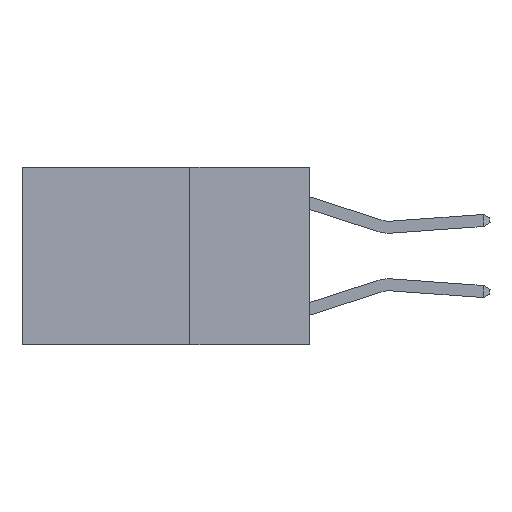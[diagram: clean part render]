
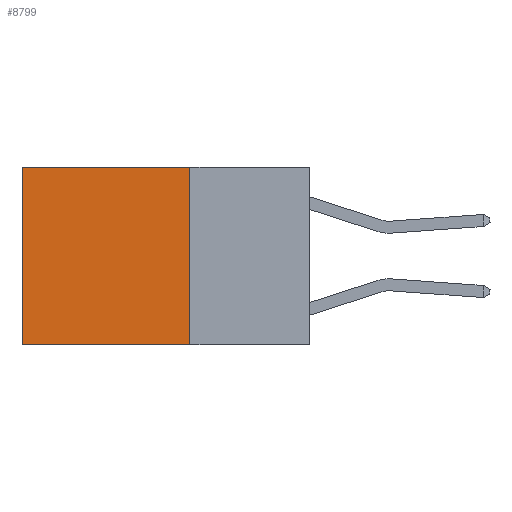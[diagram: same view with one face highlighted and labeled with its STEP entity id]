
A CAD part, left-side view. The second image highlights one B-rep face of the part: STEP entity #8799.
In plain terms, the highlighted planar face has unit normal (-1, 0, 0).
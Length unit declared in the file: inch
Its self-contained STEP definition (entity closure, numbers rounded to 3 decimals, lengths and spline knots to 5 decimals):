
#85 = ORIENTED_EDGE ( 'NONE', *, *, #1875, .F. ) ;
#963 = EDGE_CURVE ( 'NONE', #2235, #10444, #7236, .T. ) ;
#1875 = EDGE_CURVE ( 'NONE', #7877, #9755, #11947, .T. ) ;
#2063 = CARTESIAN_POINT ( 'NONE',  ( 0.2625, 0.25, 0. ) ) ;
#2235 = VERTEX_POINT ( 'NONE', #2063 ) ;
#2325 = CARTESIAN_POINT ( 'NONE',  ( 0.2625, 0.6, 0. ) ) ;
#3288 = DIRECTION ( 'NONE',  ( 0., 1., 0. ) ) ;
#3861 = AXIS2_PLACEMENT_3D ( 'NONE', #6731, #15380, #10451 ) ;
#4189 = CARTESIAN_POINT ( 'NONE',  ( 0.2625, 0.25, 0. ) ) ;
#5279 = DIRECTION ( 'NONE',  ( 0., 0., -1. ) ) ;
#5833 = DIRECTION ( 'NONE',  ( 0., 0., -1. ) ) ;
#6412 = CARTESIAN_POINT ( 'NONE',  ( 0.2625, 0.25, -0.37 ) ) ;
#6438 = CARTESIAN_POINT ( 'NONE',  ( 0.2625, 0.6, -0.37 ) ) ;
#6731 = CARTESIAN_POINT ( 'NONE',  ( 0.2625, 0.25, 0. ) ) ;
#6911 = VECTOR ( 'NONE', #3288, 39.37008 ) ;
#6963 = CARTESIAN_POINT ( 'NONE',  ( 0.2625, 0.25, -0.37 ) ) ;
#7236 = LINE ( 'NONE', #7550, #7665 ) ;
#7550 = CARTESIAN_POINT ( 'NONE',  ( 0.2625, 0.25, 0. ) ) ;
#7665 = VECTOR ( 'NONE', #8427, 39.37008 ) ;
#7877 = VERTEX_POINT ( 'NONE', #6412 ) ;
#8038 = CARTESIAN_POINT ( 'NONE',  ( 0.2625, 0.6, 0. ) ) ;
#8427 = DIRECTION ( 'NONE',  ( 0., 1., 0. ) ) ;
#8585 = EDGE_CURVE ( 'NONE', #2235, #7877, #15173, .T. ) ;
#8799 = ADVANCED_FACE ( 'NONE', ( #10532 ), #11553, .F. ) ;
#8884 = VECTOR ( 'NONE', #5279, 39.37008 ) ;
#9755 = VERTEX_POINT ( 'NONE', #6438 ) ;
#10216 = ORIENTED_EDGE ( 'NONE', *, *, #13133, .T. ) ;
#10444 = VERTEX_POINT ( 'NONE', #8038 ) ;
#10451 = DIRECTION ( 'NONE',  ( 0., 0., -1. ) ) ;
#10532 = FACE_OUTER_BOUND ( 'NONE', #14346, .T. ) ;
#10666 = ORIENTED_EDGE ( 'NONE', *, *, #8585, .F. ) ;
#11553 = PLANE ( 'NONE',  #3861 ) ;
#11769 = LINE ( 'NONE', #2325, #12956 ) ;
#11947 = LINE ( 'NONE', #6963, #6911 ) ;
#12956 = VECTOR ( 'NONE', #5833, 39.37008 ) ;
#13133 = EDGE_CURVE ( 'NONE', #10444, #9755, #11769, .T. ) ;
#13990 = ORIENTED_EDGE ( 'NONE', *, *, #963, .T. ) ;
#14346 = EDGE_LOOP ( 'NONE', ( #10216, #85, #10666, #13990 ) ) ;
#15173 = LINE ( 'NONE', #4189, #8884 ) ;
#15380 = DIRECTION ( 'NONE',  ( 1., 0., 0. ) ) ;
